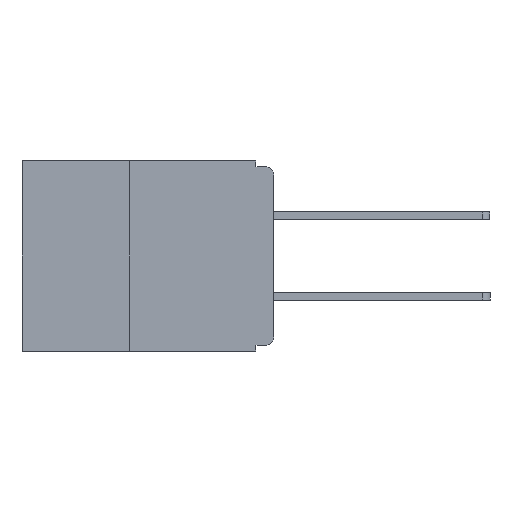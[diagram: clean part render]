
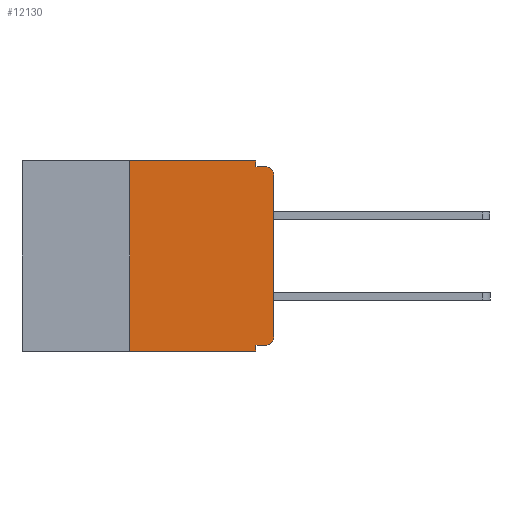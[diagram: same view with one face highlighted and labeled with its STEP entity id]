
A CAD part, left-side view. The second image highlights one B-rep face of the part: STEP entity #12130.
In plain terms, the highlighted planar face has unit normal (-1, 0, 0).
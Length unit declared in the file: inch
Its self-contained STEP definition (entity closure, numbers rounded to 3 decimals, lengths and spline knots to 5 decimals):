
#46 = VECTOR ( 'NONE', #3188, 39.37008 ) ;
#807 = CARTESIAN_POINT ( 'NONE',  ( 0., 0.25, 0. ) ) ;
#1373 = VECTOR ( 'NONE', #5241, 39.37008 ) ;
#1488 = DIRECTION ( 'NONE',  ( 0., 0., 1. ) ) ;
#1585 = ORIENTED_EDGE ( 'NONE', *, *, #6281, .F. ) ;
#1751 = AXIS2_PLACEMENT_3D ( 'NONE', #4741, #4723, #4624 ) ;
#1752 = VECTOR ( 'NONE', #10436, 39.37008 ) ;
#2015 = CARTESIAN_POINT ( 'NONE',  ( 0., 0.25, -0.33 ) ) ;
#2031 = LINE ( 'NONE', #15727, #5870 ) ;
#2184 = VERTEX_POINT ( 'NONE', #8607 ) ;
#2303 = CARTESIAN_POINT ( 'NONE',  ( 0., 0.437, 0. ) ) ;
#2558 = VERTEX_POINT ( 'NONE', #6511 ) ;
#2958 = EDGE_CURVE ( 'NONE', #6978, #18677, #4529, .T. ) ;
#3188 = DIRECTION ( 'NONE',  ( 0., -1., 0. ) ) ;
#3454 = EDGE_CURVE ( 'NONE', #8490, #2558, #8329, .T. ) ;
#3934 = ORIENTED_EDGE ( 'NONE', *, *, #16037, .T. ) ;
#3945 = CARTESIAN_POINT ( 'NONE',  ( 0., 0.015, -0.32 ) ) ;
#4529 = LINE ( 'NONE', #7926, #46 ) ;
#4624 = DIRECTION ( 'NONE',  ( 0., 0., -1. ) ) ;
#4723 = DIRECTION ( 'NONE',  ( -1., 0., 0. ) ) ;
#4741 = CARTESIAN_POINT ( 'NONE',  ( 0., 0.015, -0.305 ) ) ;
#4863 = ORIENTED_EDGE ( 'NONE', *, *, #18730, .F. ) ;
#5241 = DIRECTION ( 'NONE',  ( 0., 0., 1. ) ) ;
#5267 = LINE ( 'NONE', #7594, #17508 ) ;
#5433 = ORIENTED_EDGE ( 'NONE', *, *, #3454, .T. ) ;
#5497 = VECTOR ( 'NONE', #1488, 39.37008 ) ;
#5625 = CARTESIAN_POINT ( 'NONE',  ( 0., 0.031, -0.32 ) ) ;
#5869 = EDGE_CURVE ( 'NONE', #8490, #8531, #5267, .T. ) ;
#5870 = VECTOR ( 'NONE', #7799, 39.37008 ) ;
#6279 = ORIENTED_EDGE ( 'NONE', *, *, #12674, .F. ) ;
#6281 = EDGE_CURVE ( 'NONE', #8756, #6471, #14299, .T. ) ;
#6471 = VERTEX_POINT ( 'NONE', #807 ) ;
#6496 = CARTESIAN_POINT ( 'NONE',  ( 0., 0.437, 0. ) ) ;
#6511 = CARTESIAN_POINT ( 'NONE',  ( 0., 0., -0.305 ) ) ;
#6578 = EDGE_CURVE ( 'NONE', #13305, #18677, #17732, .T. ) ;
#6977 = EDGE_LOOP ( 'NONE', ( #3934, #20343, #11692, #7324, #6279, #1585, #14167, #4863, #10657, #5433 ) ) ;
#6978 = VERTEX_POINT ( 'NONE', #16184 ) ;
#7052 = CARTESIAN_POINT ( 'NONE',  ( 0., 0., -0.025 ) ) ;
#7232 = CARTESIAN_POINT ( 'NONE',  ( 0., 0.015, -0.01 ) ) ;
#7324 = ORIENTED_EDGE ( 'NONE', *, *, #19687, .F. ) ;
#7506 = CARTESIAN_POINT ( 'NONE',  ( 0., 0.031, -0.33 ) ) ;
#7594 = CARTESIAN_POINT ( 'NONE',  ( 0., 0., -0.32 ) ) ;
#7754 = CARTESIAN_POINT ( 'NONE',  ( 0., 0.25, -0.33 ) ) ;
#7799 = DIRECTION ( 'NONE',  ( 0., -1., 0. ) ) ;
#7926 = CARTESIAN_POINT ( 'NONE',  ( 0., 0., -0.01 ) ) ;
#8167 = DIRECTION ( 'NONE',  ( 0., 0., -1. ) ) ;
#8329 = CIRCLE ( 'NONE', #1751, 0.015 ) ;
#8490 = VERTEX_POINT ( 'NONE', #3945 ) ;
#8502 = DIRECTION ( 'NONE',  ( 0., 0., -1. ) ) ;
#8531 = VERTEX_POINT ( 'NONE', #5625 ) ;
#8607 = CARTESIAN_POINT ( 'NONE',  ( 0., 0.031, 0. ) ) ;
#8756 = VERTEX_POINT ( 'NONE', #7754 ) ;
#8931 = DIRECTION ( 'NONE',  ( -1., 0., 0. ) ) ;
#10072 = LINE ( 'NONE', #7506, #14251 ) ;
#10436 = DIRECTION ( 'NONE',  ( 0., -1., 0. ) ) ;
#10657 = ORIENTED_EDGE ( 'NONE', *, *, #5869, .F. ) ;
#11692 = ORIENTED_EDGE ( 'NONE', *, *, #2958, .F. ) ;
#12130 = ADVANCED_FACE ( 'NONE', ( #20265 ), #12924, .F. ) ;
#12460 = DIRECTION ( 'NONE',  ( 0., 1., 0. ) ) ;
#12674 = EDGE_CURVE ( 'NONE', #6471, #2184, #14654, .T. ) ;
#12869 = CARTESIAN_POINT ( 'NONE',  ( 0., 0., 0. ) ) ;
#12924 = PLANE ( 'NONE',  #14891 ) ;
#13070 = LINE ( 'NONE', #12869, #5497 ) ;
#13305 = VERTEX_POINT ( 'NONE', #7052 ) ;
#14167 = ORIENTED_EDGE ( 'NONE', *, *, #20604, .T. ) ;
#14251 = VECTOR ( 'NONE', #15454, 39.37008 ) ;
#14299 = LINE ( 'NONE', #2015, #1373 ) ;
#14654 = LINE ( 'NONE', #2303, #1752 ) ;
#14825 = CARTESIAN_POINT ( 'NONE',  ( 0., 0.031, 0. ) ) ;
#14891 = AXIS2_PLACEMENT_3D ( 'NONE', #6496, #17662, #8167 ) ;
#14955 = AXIS2_PLACEMENT_3D ( 'NONE', #18398, #8931, #19932 ) ;
#15454 = DIRECTION ( 'NONE',  ( 0., 0., -1. ) ) ;
#15727 = CARTESIAN_POINT ( 'NONE',  ( 0., 0.437, -0.33 ) ) ;
#16037 = EDGE_CURVE ( 'NONE', #2558, #13305, #13070, .T. ) ;
#16184 = CARTESIAN_POINT ( 'NONE',  ( 0., 0.031, -0.01 ) ) ;
#16422 = LINE ( 'NONE', #14825, #20047 ) ;
#16717 = CARTESIAN_POINT ( 'NONE',  ( 0., 0.031, -0.33 ) ) ;
#17508 = VECTOR ( 'NONE', #12460, 39.37008 ) ;
#17662 = DIRECTION ( 'NONE',  ( 1., 0., 0. ) ) ;
#17732 = CIRCLE ( 'NONE', #14955, 0.015 ) ;
#18398 = CARTESIAN_POINT ( 'NONE',  ( 0., 0.015, -0.025 ) ) ;
#18677 = VERTEX_POINT ( 'NONE', #7232 ) ;
#18730 = EDGE_CURVE ( 'NONE', #8531, #20376, #10072, .T. ) ;
#19687 = EDGE_CURVE ( 'NONE', #2184, #6978, #16422, .T. ) ;
#19932 = DIRECTION ( 'NONE',  ( 0., 0., -1. ) ) ;
#20047 = VECTOR ( 'NONE', #8502, 39.37008 ) ;
#20265 = FACE_OUTER_BOUND ( 'NONE', #6977, .T. ) ;
#20343 = ORIENTED_EDGE ( 'NONE', *, *, #6578, .T. ) ;
#20376 = VERTEX_POINT ( 'NONE', #16717 ) ;
#20604 = EDGE_CURVE ( 'NONE', #8756, #20376, #2031, .T. ) ;
